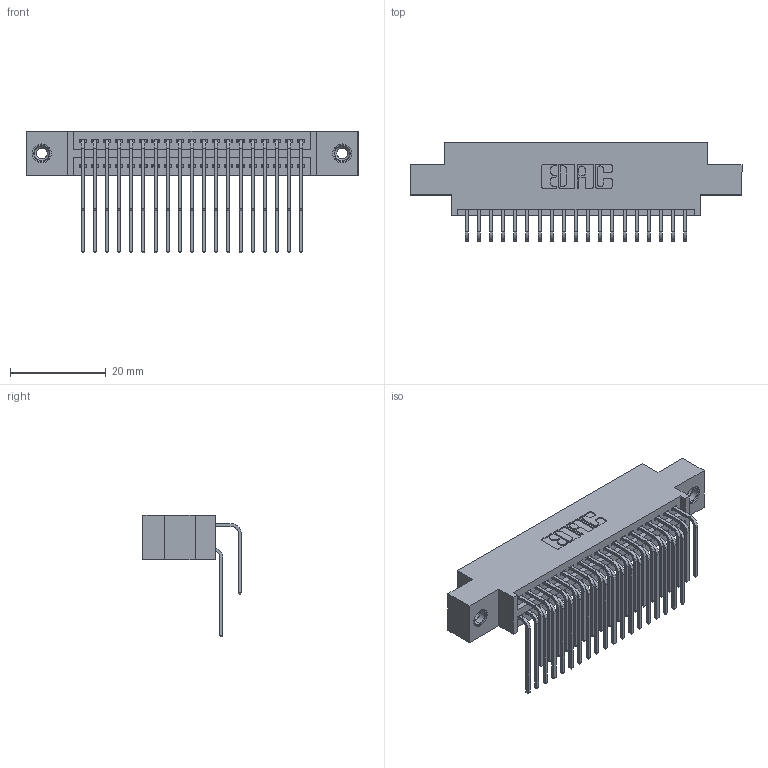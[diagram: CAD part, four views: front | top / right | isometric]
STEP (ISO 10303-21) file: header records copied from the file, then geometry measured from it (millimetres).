
FILE_DESCRIPTION (( 'STEP AP203' ), '1' );
FILE_NAME ('345-038-559-808.STEP', '2018-08-30T10:45:40', ( '' ), ( '' ), 'SwSTEP 2.0', 'SolidWorks 2016', '' );
FILE_SCHEMA (( 'CONFIG_CONTROL_DESIGN' ));
Length unit declared in the file: inch
Products named in the file (5): 345-038-559-808; 345 Part_0.170 Offset - 0.156 Dia-TI; 345-292-001_558 559 Tail - 1; 345-292-001_559 Tail - 2; 345-250-001_345-250-003-102
Assembly tree (41 placements, depth 2):
  345-038-559-808
    345 Part_0.170 Offset - 0.156 Dia-TI
    345-292-001_558 559 Tail - 1  x19
    345-292-001_559 Tail - 2  x19
    345-250-001_345-250-003-102  x2
Bounding box: 69.47 x 20.56 x 25.53 mm (x, y, z)
Volume: 6634.1 mm3; surface area: 10548.6 mm2
Topology: 41 solids, 41 shells, 2166 faces, 6379 edges, 4194 vertices
Faces by surface type: plane 1446, cylinder 704, cone 12, torus 4
Entity records: 20974 total; most frequent: CARTESIAN_POINT 3566, ORIENTED_EDGE 3442, DIRECTION 3171, EDGE_CURVE 1721, VECTOR 1453, LINE 1453, VERTEX_POINT 1140, AXIS2_PLACEMENT_3D 859
